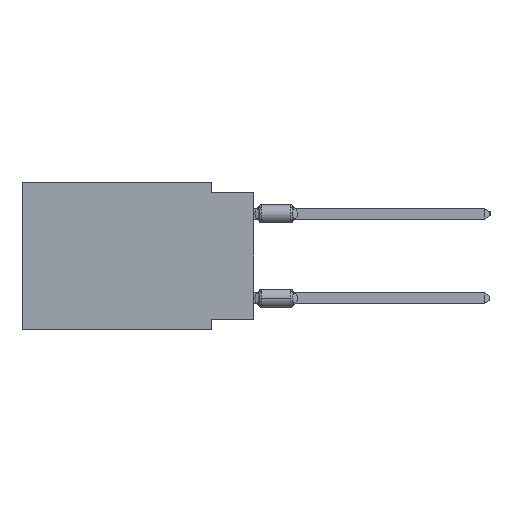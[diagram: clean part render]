
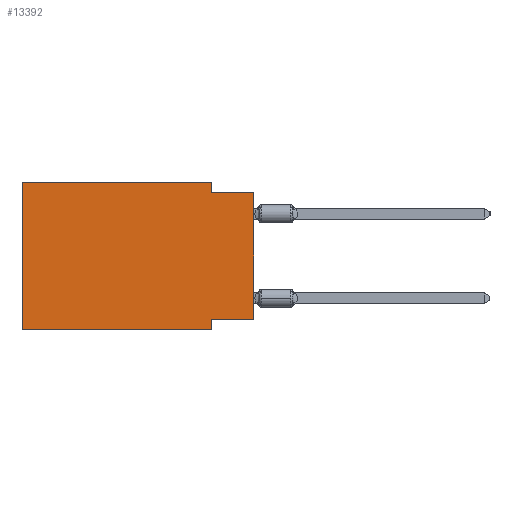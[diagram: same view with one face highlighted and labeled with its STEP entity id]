
A CAD part, left-side view. The second image highlights one B-rep face of the part: STEP entity #13392.
In plain terms, the highlighted planar face has unit normal (-1, 0, 0).
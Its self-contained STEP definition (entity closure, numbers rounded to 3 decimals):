
#1153 = EDGE_CURVE ( 'NONE', #19569, #21634, #31015, .T. ) ;
#1808 = VERTEX_POINT ( 'NONE', #48055 ) ;
#2893 = EDGE_LOOP ( 'NONE', ( #24523, #16317, #3301, #42094, #44287, #60197, #21428, #21451 ) ) ;
#3053 = CARTESIAN_POINT ( 'NONE',  ( 0., 13.97, 0. ) ) ;
#3301 = ORIENTED_EDGE ( 'NONE', *, *, #6416, .F. ) ;
#4168 = DIRECTION ( 'NONE',  ( 0., 0., 1. ) ) ;
#4643 = DIRECTION ( 'NONE',  ( 0., 1., 0. ) ) ;
#5091 = CARTESIAN_POINT ( 'NONE',  ( 0., 13.97, 0. ) ) ;
#5370 = EDGE_CURVE ( 'NONE', #17007, #1808, #29001, .T. ) ;
#6102 = EDGE_CURVE ( 'NONE', #13933, #53873, #27929, .T. ) ;
#6416 = EDGE_CURVE ( 'NONE', #12873, #19569, #41433, .T. ) ;
#7599 = EDGE_CURVE ( 'NONE', #17007, #21634, #19057, .T. ) ;
#8368 = FACE_OUTER_BOUND ( 'NONE', #2893, .T. ) ;
#9278 = DIRECTION ( 'NONE',  ( 1., 0., 0. ) ) ;
#12067 = CARTESIAN_POINT ( 'NONE',  ( 0., 13.97, -8.89 ) ) ;
#12254 = CARTESIAN_POINT ( 'NONE',  ( 0., 2.54, -8.89 ) ) ;
#12873 = VERTEX_POINT ( 'NONE', #32807 ) ;
#13392 = ADVANCED_FACE ( 'NONE', ( #8368 ), #46598, .F. ) ;
#13933 = VERTEX_POINT ( 'NONE', #12067 ) ;
#14126 = CARTESIAN_POINT ( 'NONE',  ( 0., 0., 0. ) ) ;
#15137 = LINE ( 'NONE', #28408, #48160 ) ;
#15706 = AXIS2_PLACEMENT_3D ( 'NONE', #17947, #9278, #50630 ) ;
#15959 = DIRECTION ( 'NONE',  ( 0., 0., -1. ) ) ;
#16317 = ORIENTED_EDGE ( 'NONE', *, *, #1153, .F. ) ;
#17007 = VERTEX_POINT ( 'NONE', #24358 ) ;
#17403 = CARTESIAN_POINT ( 'NONE',  ( 0., 2.54, 0. ) ) ;
#17709 = CARTESIAN_POINT ( 'NONE',  ( 0., 2.54, -8.89 ) ) ;
#17756 = VECTOR ( 'NONE', #4168, 1000. ) ;
#17947 = CARTESIAN_POINT ( 'NONE',  ( 0., 13.97, 0. ) ) ;
#19057 = LINE ( 'NONE', #14126, #50231 ) ;
#19458 = CARTESIAN_POINT ( 'NONE',  ( 0., 0., -8.255 ) ) ;
#19569 = VERTEX_POINT ( 'NONE', #38915 ) ;
#20839 = DIRECTION ( 'NONE',  ( 0., -1., 0. ) ) ;
#21428 = ORIENTED_EDGE ( 'NONE', *, *, #45786, .F. ) ;
#21451 = ORIENTED_EDGE ( 'NONE', *, *, #5370, .F. ) ;
#21634 = VERTEX_POINT ( 'NONE', #51426 ) ;
#24358 = CARTESIAN_POINT ( 'NONE',  ( 0., 0., -8.255 ) ) ;
#24523 = ORIENTED_EDGE ( 'NONE', *, *, #7599, .T. ) ;
#26075 = CARTESIAN_POINT ( 'NONE',  ( 0., 0., -0.635 ) ) ;
#26489 = VECTOR ( 'NONE', #54878, 1000. ) ;
#27929 = LINE ( 'NONE', #5091, #17756 ) ;
#28408 = CARTESIAN_POINT ( 'NONE',  ( 0., 13.97, -8.89 ) ) ;
#29001 = LINE ( 'NONE', #19458, #29493 ) ;
#29493 = VECTOR ( 'NONE', #4643, 1000. ) ;
#31015 = LINE ( 'NONE', #26075, #59545 ) ;
#32807 = CARTESIAN_POINT ( 'NONE',  ( 0., 2.54, 0. ) ) ;
#32943 = DIRECTION ( 'NONE',  ( 0., 0., 1. ) ) ;
#36376 = LINE ( 'NONE', #3053, #26489 ) ;
#37969 = VERTEX_POINT ( 'NONE', #12254 ) ;
#38915 = CARTESIAN_POINT ( 'NONE',  ( 0., 2.54, -0.635 ) ) ;
#40152 = CARTESIAN_POINT ( 'NONE',  ( 0., 13.97, 0. ) ) ;
#40445 = EDGE_CURVE ( 'NONE', #13933, #37969, #15137, .T. ) ;
#41139 = LINE ( 'NONE', #17709, #51008 ) ;
#41433 = LINE ( 'NONE', #17403, #58100 ) ;
#42094 = ORIENTED_EDGE ( 'NONE', *, *, #46683, .F. ) ;
#44287 = ORIENTED_EDGE ( 'NONE', *, *, #6102, .F. ) ;
#45786 = EDGE_CURVE ( 'NONE', #1808, #37969, #41139, .T. ) ;
#46598 = PLANE ( 'NONE',  #15706 ) ;
#46683 = EDGE_CURVE ( 'NONE', #53873, #12873, #36376, .T. ) ;
#47208 = DIRECTION ( 'NONE',  ( 0., -1., 0. ) ) ;
#48055 = CARTESIAN_POINT ( 'NONE',  ( 0., 2.54, -8.255 ) ) ;
#48160 = VECTOR ( 'NONE', #47208, 1000. ) ;
#50231 = VECTOR ( 'NONE', #32943, 1000. ) ;
#50630 = DIRECTION ( 'NONE',  ( 0., 0., -1. ) ) ;
#51008 = VECTOR ( 'NONE', #15959, 1000. ) ;
#51426 = CARTESIAN_POINT ( 'NONE',  ( 0., 0., -0.635 ) ) ;
#53873 = VERTEX_POINT ( 'NONE', #40152 ) ;
#54878 = DIRECTION ( 'NONE',  ( 0., -1., 0. ) ) ;
#58100 = VECTOR ( 'NONE', #60233, 1000. ) ;
#59545 = VECTOR ( 'NONE', #20839, 1000. ) ;
#60197 = ORIENTED_EDGE ( 'NONE', *, *, #40445, .T. ) ;
#60233 = DIRECTION ( 'NONE',  ( 0., 0., -1. ) ) ;
